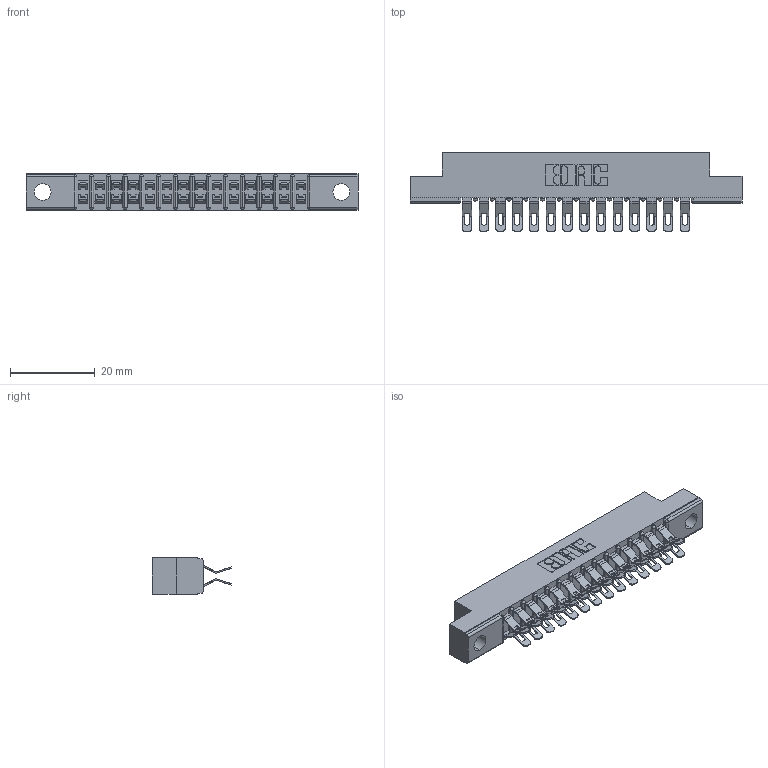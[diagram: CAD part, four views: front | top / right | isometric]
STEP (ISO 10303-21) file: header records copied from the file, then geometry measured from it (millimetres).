
FILE_DESCRIPTION (( 'STEP AP203' ), '1' );
FILE_NAME ('357-028-555-204.STEP', '2019-09-17T23:48:52', ( '' ), ( '' ), 'SwSTEP 2.0', 'SolidWorks 2016', '' );
FILE_SCHEMA (( 'CONFIG_CONTROL_DESIGN' ));
Length unit declared in the file: inch
Products named in the file (3): 357-028-555-204; 307 Part_.156 Dia Mounting Holes; 307-290-001_555
Assembly tree (29 placements, depth 2):
  357-028-555-204
    307 Part_.156 Dia Mounting Holes
    307-290-001_555  x28
Bounding box: 78.49 x 18.75 x 8.71 mm (x, y, z)
Volume: 5112.2 mm3; surface area: 8961.4 mm2
Topology: 29 solids, 29 shells, 1855 faces, 5427 edges, 3538 vertices
Faces by surface type: plane 1036, cylinder 789, sphere 30
Entity records: 16857 total; most frequent: CARTESIAN_POINT 2776, ORIENTED_EDGE 2748, DIRECTION 2730, EDGE_CURVE 1374, VECTOR 1038, LINE 1038, VERTEX_POINT 892, AXIS2_PLACEMENT_3D 846
